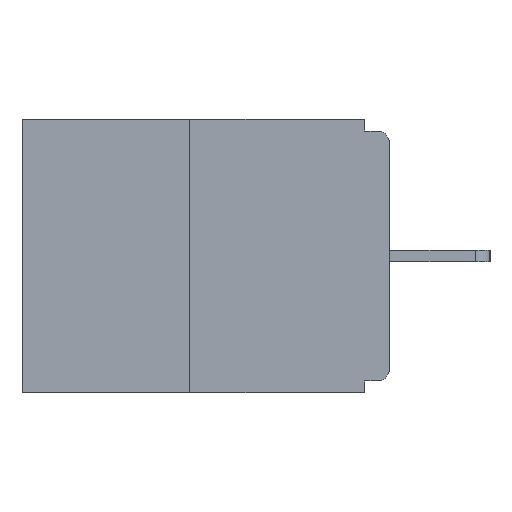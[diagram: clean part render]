
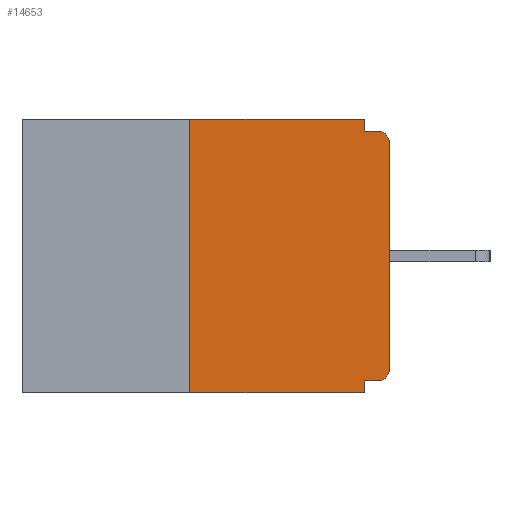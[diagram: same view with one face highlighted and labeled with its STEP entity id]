
A CAD part, left-side view. The second image highlights one B-rep face of the part: STEP entity #14653.
In plain terms, the highlighted planar face has unit normal (-1, 0, 0).
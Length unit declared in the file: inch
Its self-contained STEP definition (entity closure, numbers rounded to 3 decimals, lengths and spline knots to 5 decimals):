
#182 = CARTESIAN_POINT ( 'NONE',  ( 0., 0.031, 0. ) ) ;
#212 = VERTEX_POINT ( 'NONE', #182 ) ;
#229 = DIRECTION ( 'NONE',  ( 0., -1., 0. ) ) ;
#305 = AXIS2_PLACEMENT_3D ( 'NONE', #17010, #5704, #4245 ) ;
#333 = ORIENTED_EDGE ( 'NONE', *, *, #3054, .F. ) ;
#507 = CARTESIAN_POINT ( 'NONE',  ( 0., 0.015, -0.313 ) ) ;
#710 = AXIS2_PLACEMENT_3D ( 'NONE', #11319, #16847, #4430 ) ;
#1134 = LINE ( 'NONE', #10632, #6931 ) ;
#1292 = CARTESIAN_POINT ( 'NONE',  ( 0., 0.25, 0. ) ) ;
#1672 = DIRECTION ( 'NONE',  ( 0., 0., -1. ) ) ;
#2448 = VERTEX_POINT ( 'NONE', #2792 ) ;
#2545 = VERTEX_POINT ( 'NONE', #7035 ) ;
#2792 = CARTESIAN_POINT ( 'NONE',  ( 0., 0.031, -0.015 ) ) ;
#2798 = ORIENTED_EDGE ( 'NONE', *, *, #12293, .F. ) ;
#2860 = VECTOR ( 'NONE', #1672, 39.37008 ) ;
#3054 = EDGE_CURVE ( 'NONE', #13197, #212, #16887, .T. ) ;
#3203 = DIRECTION ( 'NONE',  ( 0., -1., 0. ) ) ;
#3461 = CARTESIAN_POINT ( 'NONE',  ( 0., 0.25, -0.343 ) ) ;
#3519 = EDGE_CURVE ( 'NONE', #2448, #17564, #7086, .T. ) ;
#3637 = DIRECTION ( 'NONE',  ( 0., 0., 1. ) ) ;
#3746 = DIRECTION ( 'NONE',  ( 0., 0., -1. ) ) ;
#4043 = VECTOR ( 'NONE', #12429, 39.37008 ) ;
#4112 = CARTESIAN_POINT ( 'NONE',  ( 0., 0.015, -0.015 ) ) ;
#4245 = DIRECTION ( 'NONE',  ( 0., 0., -1. ) ) ;
#4330 = FACE_OUTER_BOUND ( 'NONE', #8065, .T. ) ;
#4430 = DIRECTION ( 'NONE',  ( 0., 0., -1. ) ) ;
#4681 = CARTESIAN_POINT ( 'NONE',  ( 0., 0.015, -0.328 ) ) ;
#4856 = VECTOR ( 'NONE', #12965, 39.37008 ) ;
#5326 = VERTEX_POINT ( 'NONE', #4681 ) ;
#5704 = DIRECTION ( 'NONE',  ( 1., 0., 0. ) ) ;
#5708 = EDGE_CURVE ( 'NONE', #5326, #9642, #11855, .T. ) ;
#5832 = EDGE_CURVE ( 'NONE', #9642, #12909, #1134, .T. ) ;
#6899 = CARTESIAN_POINT ( 'NONE',  ( 0., 0.031, -0.343 ) ) ;
#6931 = VECTOR ( 'NONE', #9450, 39.37008 ) ;
#7035 = CARTESIAN_POINT ( 'NONE',  ( 0., 0.031, -0.328 ) ) ;
#7086 = LINE ( 'NONE', #14060, #16524 ) ;
#7210 = VERTEX_POINT ( 'NONE', #3461 ) ;
#7730 = ORIENTED_EDGE ( 'NONE', *, *, #3519, .F. ) ;
#7743 = EDGE_CURVE ( 'NONE', #5326, #2545, #15683, .T. ) ;
#7785 = CARTESIAN_POINT ( 'NONE',  ( 0., 0.25, 0. ) ) ;
#7965 = CARTESIAN_POINT ( 'NONE',  ( 0., 0.46, -0.343 ) ) ;
#8065 = EDGE_LOOP ( 'NONE', ( #333, #2798, #14051, #14349, #16528, #12112, #17698, #14095, #7730, #16289 ) ) ;
#8090 = LINE ( 'NONE', #17694, #10700 ) ;
#8107 = VECTOR ( 'NONE', #3637, 39.37008 ) ;
#8618 = LINE ( 'NONE', #6899, #2860 ) ;
#8691 = EDGE_CURVE ( 'NONE', #12909, #17564, #17752, .T. ) ;
#8827 = DIRECTION ( 'NONE',  ( -1., 0., 0. ) ) ;
#9450 = DIRECTION ( 'NONE',  ( 0., 0., 1. ) ) ;
#9642 = VERTEX_POINT ( 'NONE', #10612 ) ;
#10558 = VECTOR ( 'NONE', #3203, 39.37008 ) ;
#10612 = CARTESIAN_POINT ( 'NONE',  ( 0., 0., -0.313 ) ) ;
#10632 = CARTESIAN_POINT ( 'NONE',  ( 0., 0., 0. ) ) ;
#10700 = VECTOR ( 'NONE', #3746, 39.37008 ) ;
#10865 = CARTESIAN_POINT ( 'NONE',  ( 0., 0.031, -0.343 ) ) ;
#11128 = EDGE_CURVE ( 'NONE', #2545, #16156, #8618, .T. ) ;
#11231 = PLANE ( 'NONE',  #305 ) ;
#11274 = CARTESIAN_POINT ( 'NONE',  ( 0., 0.46, 0. ) ) ;
#11319 = CARTESIAN_POINT ( 'NONE',  ( 0., 0.015, -0.03 ) ) ;
#11855 = CIRCLE ( 'NONE', #17043, 0.015 ) ;
#12112 = ORIENTED_EDGE ( 'NONE', *, *, #5708, .T. ) ;
#12148 = EDGE_CURVE ( 'NONE', #212, #2448, #8090, .T. ) ;
#12293 = EDGE_CURVE ( 'NONE', #7210, #13197, #15780, .T. ) ;
#12429 = DIRECTION ( 'NONE',  ( 0., -1., 0. ) ) ;
#12909 = VERTEX_POINT ( 'NONE', #16861 ) ;
#12965 = DIRECTION ( 'NONE',  ( 0., 1., 0. ) ) ;
#13060 = CARTESIAN_POINT ( 'NONE',  ( 0., 0., -0.328 ) ) ;
#13197 = VERTEX_POINT ( 'NONE', #1292 ) ;
#14051 = ORIENTED_EDGE ( 'NONE', *, *, #14538, .T. ) ;
#14060 = CARTESIAN_POINT ( 'NONE',  ( 0., 0., -0.015 ) ) ;
#14095 = ORIENTED_EDGE ( 'NONE', *, *, #8691, .T. ) ;
#14349 = ORIENTED_EDGE ( 'NONE', *, *, #11128, .F. ) ;
#14538 = EDGE_CURVE ( 'NONE', #7210, #16156, #17840, .T. ) ;
#14653 = ADVANCED_FACE ( 'NONE', ( #4330 ), #11231, .F. ) ;
#15683 = LINE ( 'NONE', #13060, #4856 ) ;
#15780 = LINE ( 'NONE', #7785, #8107 ) ;
#16156 = VERTEX_POINT ( 'NONE', #10865 ) ;
#16289 = ORIENTED_EDGE ( 'NONE', *, *, #12148, .F. ) ;
#16524 = VECTOR ( 'NONE', #229, 39.37008 ) ;
#16528 = ORIENTED_EDGE ( 'NONE', *, *, #7743, .F. ) ;
#16847 = DIRECTION ( 'NONE',  ( -1., 0., 0. ) ) ;
#16861 = CARTESIAN_POINT ( 'NONE',  ( 0., 0., -0.03 ) ) ;
#16887 = LINE ( 'NONE', #11274, #10558 ) ;
#17010 = CARTESIAN_POINT ( 'NONE',  ( 0., 0.46, 0. ) ) ;
#17043 = AXIS2_PLACEMENT_3D ( 'NONE', #507, #8827, #17422 ) ;
#17422 = DIRECTION ( 'NONE',  ( 0., 0., -1. ) ) ;
#17564 = VERTEX_POINT ( 'NONE', #4112 ) ;
#17694 = CARTESIAN_POINT ( 'NONE',  ( 0., 0.031, 0. ) ) ;
#17698 = ORIENTED_EDGE ( 'NONE', *, *, #5832, .T. ) ;
#17752 = CIRCLE ( 'NONE', #710, 0.015 ) ;
#17840 = LINE ( 'NONE', #7965, #4043 ) ;
